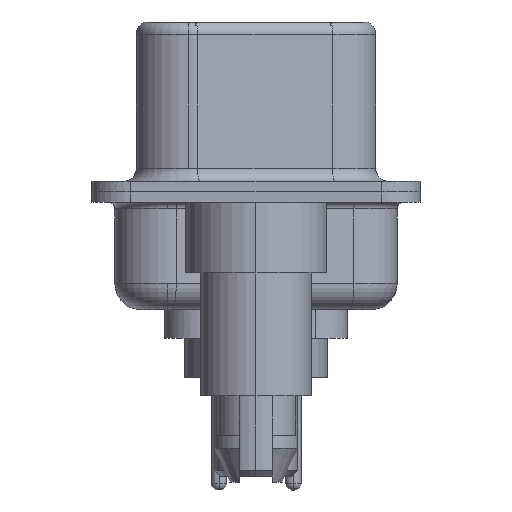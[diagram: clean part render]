
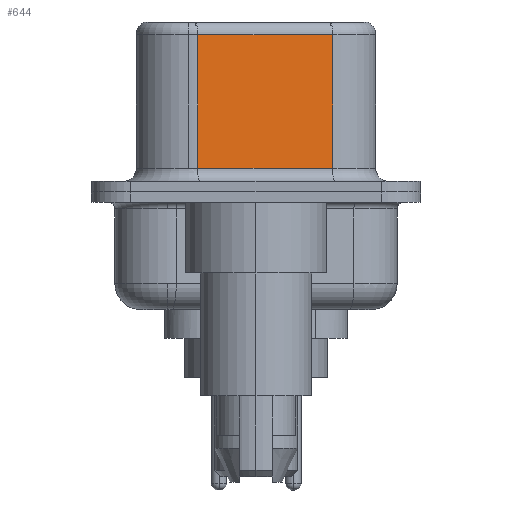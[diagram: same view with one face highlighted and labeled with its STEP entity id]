
A CAD part, left-side view. The second image highlights one B-rep face of the part: STEP entity #644.
In plain terms, the highlighted planar face has unit normal (-0.985, -0.174, 0).
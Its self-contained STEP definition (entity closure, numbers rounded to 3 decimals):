
#644 = ADVANCED_FACE ( 'NONE', ( #12807 ), #5241, .F. ) ;
#1211 = ORIENTED_EDGE ( 'NONE', *, *, #5038, .T. ) ;
#1449 = VERTEX_POINT ( 'NONE', #20764 ) ;
#2475 = CARTESIAN_POINT ( 'NONE',  ( 3.67, 2.233, 6.52 ) ) ;
#2884 = VERTEX_POINT ( 'NONE', #7510 ) ;
#3145 = CARTESIAN_POINT ( 'NONE',  ( 3.67, 2.233, 0.9 ) ) ;
#3212 = LINE ( 'NONE', #2475, #11919 ) ;
#5038 = EDGE_CURVE ( 'NONE', #2884, #10691, #5052, .T. ) ;
#5052 = LINE ( 'NONE', #12029, #14259 ) ;
#5241 = PLANE ( 'NONE',  #18649 ) ;
#6085 = DIRECTION ( 'NONE',  ( 0.985, 0.174, 0. ) ) ;
#6510 = CARTESIAN_POINT ( 'NONE',  ( 3.67, 2.233, 6.02 ) ) ;
#6746 = CARTESIAN_POINT ( 'NONE',  ( 4.58, -2.927, 6.52 ) ) ;
#6853 = CARTESIAN_POINT ( 'NONE',  ( 4.58, -2.927, 6.52 ) ) ;
#7510 = CARTESIAN_POINT ( 'NONE',  ( 4.58, -2.927, 6.02 ) ) ;
#7998 = EDGE_CURVE ( 'NONE', #21345, #1449, #18825, .T. ) ;
#8521 = DIRECTION ( 'NONE',  ( 0., 0., -1. ) ) ;
#9402 = DIRECTION ( 'NONE',  ( 0., 0., -1. ) ) ;
#9484 = DIRECTION ( 'NONE',  ( 0.174, -0.985, 0. ) ) ;
#9689 = VECTOR ( 'NONE', #9484, 1000. ) ;
#10691 = VERTEX_POINT ( 'NONE', #6510 ) ;
#10823 = VECTOR ( 'NONE', #8521, 1000. ) ;
#11919 = VECTOR ( 'NONE', #9402, 1000. ) ;
#12029 = CARTESIAN_POINT ( 'NONE',  ( 4.58, -2.927, 6.02 ) ) ;
#12807 = FACE_OUTER_BOUND ( 'NONE', #21859, .T. ) ;
#14101 = ORIENTED_EDGE ( 'NONE', *, *, #14545, .T. ) ;
#14259 = VECTOR ( 'NONE', #21421, 1000. ) ;
#14545 = EDGE_CURVE ( 'NONE', #10691, #21345, #3212, .T. ) ;
#14894 = ORIENTED_EDGE ( 'NONE', *, *, #7998, .T. ) ;
#15391 = EDGE_CURVE ( 'NONE', #2884, #1449, #19976, .T. ) ;
#17267 = ORIENTED_EDGE ( 'NONE', *, *, #15391, .F. ) ;
#18053 = CARTESIAN_POINT ( 'NONE',  ( 4.58, -2.927, 0.9 ) ) ;
#18649 = AXIS2_PLACEMENT_3D ( 'NONE', #6853, #6085, #22116 ) ;
#18825 = LINE ( 'NONE', #18053, #9689 ) ;
#19976 = LINE ( 'NONE', #6746, #10823 ) ;
#20764 = CARTESIAN_POINT ( 'NONE',  ( 4.58, -2.927, 0.9 ) ) ;
#21345 = VERTEX_POINT ( 'NONE', #3145 ) ;
#21421 = DIRECTION ( 'NONE',  ( -0.174, 0.985, 0. ) ) ;
#21859 = EDGE_LOOP ( 'NONE', ( #17267, #1211, #14101, #14894 ) ) ;
#22116 = DIRECTION ( 'NONE',  ( -0.174, 0.985, 0. ) ) ;
